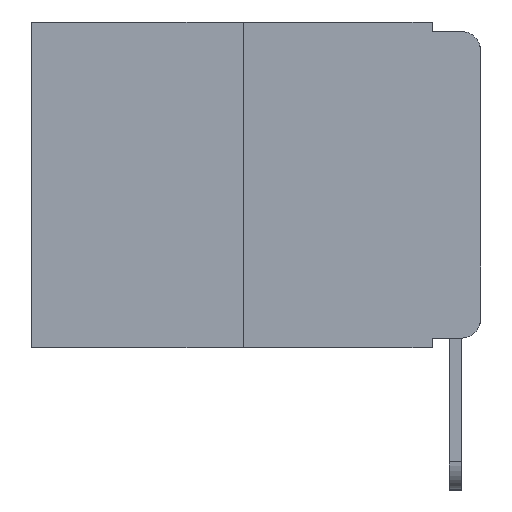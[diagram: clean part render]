
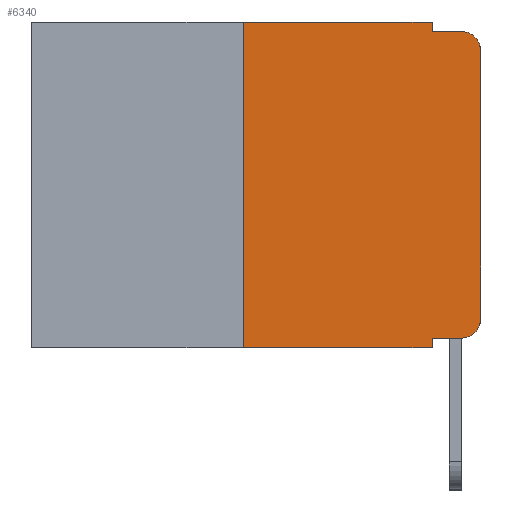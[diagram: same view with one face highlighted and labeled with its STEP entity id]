
A CAD part, left-side view. The second image highlights one B-rep face of the part: STEP entity #6340.
In plain terms, the highlighted planar face has unit normal (-1, 0, 0).
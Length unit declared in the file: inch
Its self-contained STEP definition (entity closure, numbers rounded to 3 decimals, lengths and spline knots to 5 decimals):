
#21 = DIRECTION ( 'NONE',  ( 0., -1., 0. ) ) ;
#482 = VECTOR ( 'NONE', #9780, 39.37008 ) ;
#650 = CARTESIAN_POINT ( 'NONE',  ( 0., 0.02, -0.313 ) ) ;
#747 = EDGE_CURVE ( 'NONE', #11738, #7103, #11806, .T. ) ;
#1058 = CARTESIAN_POINT ( 'NONE',  ( 0., 0.02, -0.03 ) ) ;
#1139 = DIRECTION ( 'NONE',  ( 0., -1., 0. ) ) ;
#1325 = LINE ( 'NONE', #4334, #4603 ) ;
#1328 = ORIENTED_EDGE ( 'NONE', *, *, #2847, .F. ) ;
#1336 = CARTESIAN_POINT ( 'NONE',  ( 0., 0.051, 0. ) ) ;
#1443 = VERTEX_POINT ( 'NONE', #5786 ) ;
#1519 = VERTEX_POINT ( 'NONE', #8246 ) ;
#1565 = CARTESIAN_POINT ( 'NONE',  ( 0., 0.02, -0.333 ) ) ;
#1778 = DIRECTION ( 'NONE',  ( 0., 0., -1. ) ) ;
#1897 = DIRECTION ( 'NONE',  ( 1., 0., 0. ) ) ;
#2090 = DIRECTION ( 'NONE',  ( 0., 0., 1. ) ) ;
#2160 = CARTESIAN_POINT ( 'NONE',  ( 0., 0.25, -0.343 ) ) ;
#2354 = VECTOR ( 'NONE', #2090, 39.37008 ) ;
#2704 = AXIS2_PLACEMENT_3D ( 'NONE', #1058, #11078, #4867 ) ;
#2787 = EDGE_CURVE ( 'NONE', #1519, #12649, #3399, .T. ) ;
#2847 = EDGE_CURVE ( 'NONE', #5427, #8761, #8675, .T. ) ;
#3002 = VECTOR ( 'NONE', #4070, 39.37008 ) ;
#3234 = VERTEX_POINT ( 'NONE', #9967 ) ;
#3237 = ORIENTED_EDGE ( 'NONE', *, *, #747, .F. ) ;
#3399 = LINE ( 'NONE', #10563, #5602 ) ;
#3420 = EDGE_CURVE ( 'NONE', #10127, #1443, #8488, .T. ) ;
#3530 = LINE ( 'NONE', #11759, #8791 ) ;
#4070 = DIRECTION ( 'NONE',  ( 0., 0., -1. ) ) ;
#4144 = CARTESIAN_POINT ( 'NONE',  ( 0., 0., 0. ) ) ;
#4334 = CARTESIAN_POINT ( 'NONE',  ( 0., 0.473, -0.343 ) ) ;
#4377 = VECTOR ( 'NONE', #11447, 39.37008 ) ;
#4459 = ORIENTED_EDGE ( 'NONE', *, *, #9548, .F. ) ;
#4603 = VECTOR ( 'NONE', #12677, 39.37008 ) ;
#4710 = CARTESIAN_POINT ( 'NONE',  ( 0., 0.051, 0. ) ) ;
#4867 = DIRECTION ( 'NONE',  ( 0., 0., -1. ) ) ;
#5118 = CARTESIAN_POINT ( 'NONE',  ( 0., 0.051, 0. ) ) ;
#5427 = VERTEX_POINT ( 'NONE', #2160 ) ;
#5602 = VECTOR ( 'NONE', #6677, 39.37008 ) ;
#5786 = CARTESIAN_POINT ( 'NONE',  ( 0., 0.02, -0.01 ) ) ;
#6193 = CARTESIAN_POINT ( 'NONE',  ( 0., 0.473, 0. ) ) ;
#6340 = ADVANCED_FACE ( 'NONE', ( #12263 ), #13408, .F. ) ;
#6411 = ORIENTED_EDGE ( 'NONE', *, *, #3420, .T. ) ;
#6532 = CARTESIAN_POINT ( 'NONE',  ( 0., 0.473, 0. ) ) ;
#6677 = DIRECTION ( 'NONE',  ( 0., -1., 0. ) ) ;
#7029 = VECTOR ( 'NONE', #21, 39.37008 ) ;
#7048 = CARTESIAN_POINT ( 'NONE',  ( 0., 0., -0.313 ) ) ;
#7103 = VERTEX_POINT ( 'NONE', #12940 ) ;
#7163 = LINE ( 'NONE', #4144, #4377 ) ;
#7190 = CIRCLE ( 'NONE', #13075, 0.02 ) ;
#7472 = CARTESIAN_POINT ( 'NONE',  ( 0., 0.25, 0. ) ) ;
#8001 = EDGE_LOOP ( 'NONE', ( #13334, #6411, #4459, #3237, #8049, #1328, #8351, #12710, #11622, #12873 ) ) ;
#8049 = ORIENTED_EDGE ( 'NONE', *, *, #8322, .F. ) ;
#8167 = DIRECTION ( 'NONE',  ( -1., 0., 0. ) ) ;
#8232 = DIRECTION ( 'NONE',  ( 0., 0., -1. ) ) ;
#8246 = CARTESIAN_POINT ( 'NONE',  ( 0., 0.051, -0.333 ) ) ;
#8322 = EDGE_CURVE ( 'NONE', #8761, #11738, #9805, .T. ) ;
#8351 = ORIENTED_EDGE ( 'NONE', *, *, #12278, .T. ) ;
#8416 = CARTESIAN_POINT ( 'NONE',  ( 0., 0.25, 0. ) ) ;
#8488 = CIRCLE ( 'NONE', #2704, 0.02 ) ;
#8637 = LINE ( 'NONE', #5118, #3002 ) ;
#8658 = EDGE_CURVE ( 'NONE', #1519, #3234, #8637, .T. ) ;
#8675 = LINE ( 'NONE', #7472, #2354 ) ;
#8761 = VERTEX_POINT ( 'NONE', #8416 ) ;
#8791 = VECTOR ( 'NONE', #1139, 39.37008 ) ;
#9164 = VERTEX_POINT ( 'NONE', #7048 ) ;
#9236 = EDGE_CURVE ( 'NONE', #12649, #9164, #7190, .T. ) ;
#9254 = CARTESIAN_POINT ( 'NONE',  ( 0., 0., -0.03 ) ) ;
#9548 = EDGE_CURVE ( 'NONE', #7103, #1443, #3530, .T. ) ;
#9646 = AXIS2_PLACEMENT_3D ( 'NONE', #6193, #1897, #8232 ) ;
#9780 = DIRECTION ( 'NONE',  ( 0., 0., -1. ) ) ;
#9805 = LINE ( 'NONE', #6532, #7029 ) ;
#9967 = CARTESIAN_POINT ( 'NONE',  ( 0., 0.051, -0.343 ) ) ;
#10127 = VERTEX_POINT ( 'NONE', #9254 ) ;
#10207 = EDGE_CURVE ( 'NONE', #9164, #10127, #7163, .T. ) ;
#10563 = CARTESIAN_POINT ( 'NONE',  ( 0., 0.051, -0.333 ) ) ;
#11078 = DIRECTION ( 'NONE',  ( -1., 0., 0. ) ) ;
#11447 = DIRECTION ( 'NONE',  ( 0., 0., 1. ) ) ;
#11622 = ORIENTED_EDGE ( 'NONE', *, *, #2787, .T. ) ;
#11738 = VERTEX_POINT ( 'NONE', #4710 ) ;
#11759 = CARTESIAN_POINT ( 'NONE',  ( 0., 0.051, -0.01 ) ) ;
#11806 = LINE ( 'NONE', #1336, #482 ) ;
#12263 = FACE_OUTER_BOUND ( 'NONE', #8001, .T. ) ;
#12278 = EDGE_CURVE ( 'NONE', #5427, #3234, #1325, .T. ) ;
#12649 = VERTEX_POINT ( 'NONE', #1565 ) ;
#12677 = DIRECTION ( 'NONE',  ( 0., -1., 0. ) ) ;
#12710 = ORIENTED_EDGE ( 'NONE', *, *, #8658, .F. ) ;
#12873 = ORIENTED_EDGE ( 'NONE', *, *, #9236, .T. ) ;
#12940 = CARTESIAN_POINT ( 'NONE',  ( 0., 0.051, -0.01 ) ) ;
#13075 = AXIS2_PLACEMENT_3D ( 'NONE', #650, #8167, #1778 ) ;
#13334 = ORIENTED_EDGE ( 'NONE', *, *, #10207, .T. ) ;
#13408 = PLANE ( 'NONE',  #9646 ) ;
